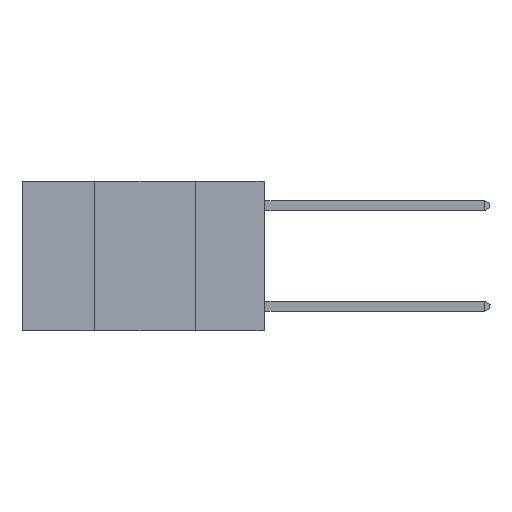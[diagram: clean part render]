
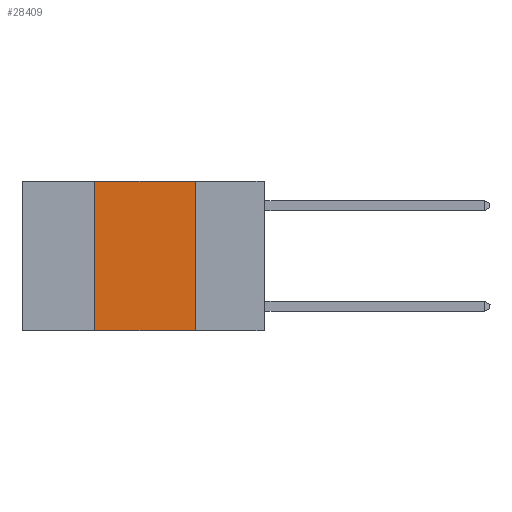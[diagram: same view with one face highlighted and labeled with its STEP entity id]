
A CAD part, left-side view. The second image highlights one B-rep face of the part: STEP entity #28409.
In plain terms, the highlighted planar face has unit normal (-1, 0, 0).
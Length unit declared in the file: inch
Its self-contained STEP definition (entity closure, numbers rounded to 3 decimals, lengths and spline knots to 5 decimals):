
#39 = CARTESIAN_POINT ( 'NONE',  ( 0., 0.6, 0. ) ) ;
#284 = ORIENTED_EDGE ( 'NONE', *, *, #12445, .F. ) ;
#372 = DIRECTION ( 'NONE',  ( 0., -1., 0. ) ) ;
#1245 = PLANE ( 'NONE',  #25841 ) ;
#1886 = EDGE_CURVE ( 'NONE', #21982, #18614, #27758, .T. ) ;
#3989 = CARTESIAN_POINT ( 'NONE',  ( 0., 0.17, 0. ) ) ;
#5738 = CARTESIAN_POINT ( 'NONE',  ( 0., 0.42, 0. ) ) ;
#5788 = DIRECTION ( 'NONE',  ( 0., 0., -1. ) ) ;
#5868 = DIRECTION ( 'NONE',  ( 0., 0., 1. ) ) ;
#6577 = EDGE_LOOP ( 'NONE', ( #16903, #22853, #284, #18316 ) ) ;
#9788 = VECTOR ( 'NONE', #13581, 39.37008 ) ;
#9833 = VERTEX_POINT ( 'NONE', #3989 ) ;
#10207 = LINE ( 'NONE', #21682, #15492 ) ;
#11724 = CARTESIAN_POINT ( 'NONE',  ( 0., 0.6, -0.37 ) ) ;
#12052 = EDGE_CURVE ( 'NONE', #22079, #9833, #15072, .T. ) ;
#12310 = CARTESIAN_POINT ( 'NONE',  ( 0., 0.17, -0.37 ) ) ;
#12445 = EDGE_CURVE ( 'NONE', #21982, #22079, #17167, .T. ) ;
#13581 = DIRECTION ( 'NONE',  ( 0., -1., 0. ) ) ;
#14837 = CARTESIAN_POINT ( 'NONE',  ( 0., 0.42, 0. ) ) ;
#15072 = LINE ( 'NONE', #39, #9788 ) ;
#15148 = VECTOR ( 'NONE', #372, 39.37008 ) ;
#15492 = VECTOR ( 'NONE', #17282, 39.37008 ) ;
#16467 = VECTOR ( 'NONE', #5868, 39.37008 ) ;
#16903 = ORIENTED_EDGE ( 'NONE', *, *, #26001, .F. ) ;
#17031 = CARTESIAN_POINT ( 'NONE',  ( 0., 0.6, 0. ) ) ;
#17167 = LINE ( 'NONE', #14837, #16467 ) ;
#17282 = DIRECTION ( 'NONE',  ( 0., 0., -1. ) ) ;
#18316 = ORIENTED_EDGE ( 'NONE', *, *, #1886, .T. ) ;
#18614 = VERTEX_POINT ( 'NONE', #12310 ) ;
#18926 = CARTESIAN_POINT ( 'NONE',  ( 0., 0.42, -0.37 ) ) ;
#19264 = DIRECTION ( 'NONE',  ( 1., 0., 0. ) ) ;
#21682 = CARTESIAN_POINT ( 'NONE',  ( 0., 0.17, 0. ) ) ;
#21982 = VERTEX_POINT ( 'NONE', #18926 ) ;
#22079 = VERTEX_POINT ( 'NONE', #5738 ) ;
#22853 = ORIENTED_EDGE ( 'NONE', *, *, #12052, .F. ) ;
#23053 = FACE_OUTER_BOUND ( 'NONE', #6577, .T. ) ;
#25841 = AXIS2_PLACEMENT_3D ( 'NONE', #17031, #19264, #5788 ) ;
#26001 = EDGE_CURVE ( 'NONE', #9833, #18614, #10207, .T. ) ;
#27758 = LINE ( 'NONE', #11724, #15148 ) ;
#28409 = ADVANCED_FACE ( 'NONE', ( #23053 ), #1245, .F. ) ;
